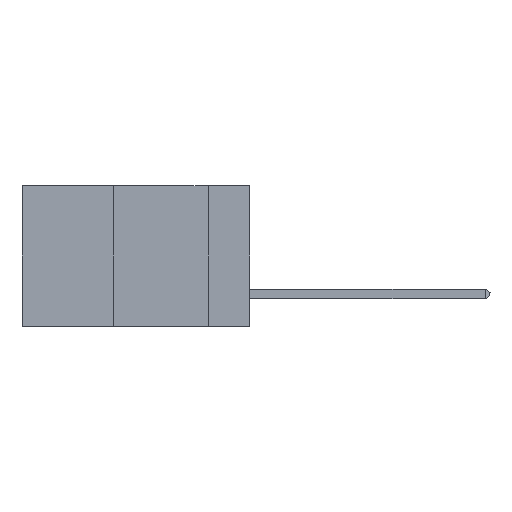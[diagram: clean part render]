
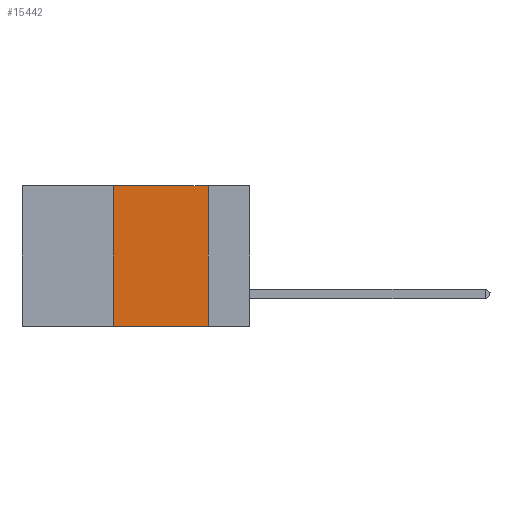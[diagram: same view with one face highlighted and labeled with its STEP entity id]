
A CAD part, left-side view. The second image highlights one B-rep face of the part: STEP entity #15442.
In plain terms, the highlighted planar face has unit normal (-1, 0, 0).
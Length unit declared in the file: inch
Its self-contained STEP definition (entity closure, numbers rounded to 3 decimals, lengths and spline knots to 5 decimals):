
#267 = CARTESIAN_POINT ( 'NONE',  ( 0., 0.6, 0. ) ) ;
#494 = CARTESIAN_POINT ( 'NONE',  ( 0., 0.11, 0. ) ) ;
#1270 = FACE_OUTER_BOUND ( 'NONE', #9840, .T. ) ;
#4076 = VERTEX_POINT ( 'NONE', #494 ) ;
#4425 = VERTEX_POINT ( 'NONE', #6058 ) ;
#4610 = ORIENTED_EDGE ( 'NONE', *, *, #15771, .T. ) ;
#4848 = CARTESIAN_POINT ( 'NONE',  ( 0., 0.6, 0. ) ) ;
#5200 = LINE ( 'NONE', #19958, #11150 ) ;
#6058 = CARTESIAN_POINT ( 'NONE',  ( 0., 0.36, 0. ) ) ;
#6644 = DIRECTION ( 'NONE',  ( 0., 0., 1. ) ) ;
#6716 = DIRECTION ( 'NONE',  ( 0., -1., 0. ) ) ;
#8573 = DIRECTION ( 'NONE',  ( 0., 0., -1. ) ) ;
#9086 = EDGE_CURVE ( 'NONE', #4076, #26662, #12177, .T. ) ;
#9840 = EDGE_LOOP ( 'NONE', ( #13872, #26731, #11516, #4610 ) ) ;
#11150 = VECTOR ( 'NONE', #24250, 39.37008 ) ;
#11516 = ORIENTED_EDGE ( 'NONE', *, *, #16908, .F. ) ;
#12177 = LINE ( 'NONE', #19295, #22432 ) ;
#12764 = VECTOR ( 'NONE', #6716, 39.37008 ) ;
#13872 = ORIENTED_EDGE ( 'NONE', *, *, #9086, .F. ) ;
#14375 = AXIS2_PLACEMENT_3D ( 'NONE', #267, #16925, #8573 ) ;
#15264 = CARTESIAN_POINT ( 'NONE',  ( 0., 0.36, 0. ) ) ;
#15442 = ADVANCED_FACE ( 'NONE', ( #1270 ), #24940, .F. ) ;
#15771 = EDGE_CURVE ( 'NONE', #15920, #26662, #5200, .T. ) ;
#15920 = VERTEX_POINT ( 'NONE', #26847 ) ;
#16908 = EDGE_CURVE ( 'NONE', #15920, #4425, #17355, .T. ) ;
#16925 = DIRECTION ( 'NONE',  ( 1., 0., 0. ) ) ;
#17355 = LINE ( 'NONE', #15264, #18708 ) ;
#17393 = LINE ( 'NONE', #4848, #12764 ) ;
#18708 = VECTOR ( 'NONE', #6644, 39.37008 ) ;
#19295 = CARTESIAN_POINT ( 'NONE',  ( 0., 0.11, 0. ) ) ;
#19958 = CARTESIAN_POINT ( 'NONE',  ( 0., 0.6, -0.37 ) ) ;
#20555 = CARTESIAN_POINT ( 'NONE',  ( 0., 0.11, -0.37 ) ) ;
#21956 = EDGE_CURVE ( 'NONE', #4425, #4076, #17393, .T. ) ;
#22432 = VECTOR ( 'NONE', #26129, 39.37008 ) ;
#24250 = DIRECTION ( 'NONE',  ( 0., -1., 0. ) ) ;
#24940 = PLANE ( 'NONE',  #14375 ) ;
#26129 = DIRECTION ( 'NONE',  ( 0., 0., -1. ) ) ;
#26662 = VERTEX_POINT ( 'NONE', #20555 ) ;
#26731 = ORIENTED_EDGE ( 'NONE', *, *, #21956, .F. ) ;
#26847 = CARTESIAN_POINT ( 'NONE',  ( 0., 0.36, -0.37 ) ) ;
